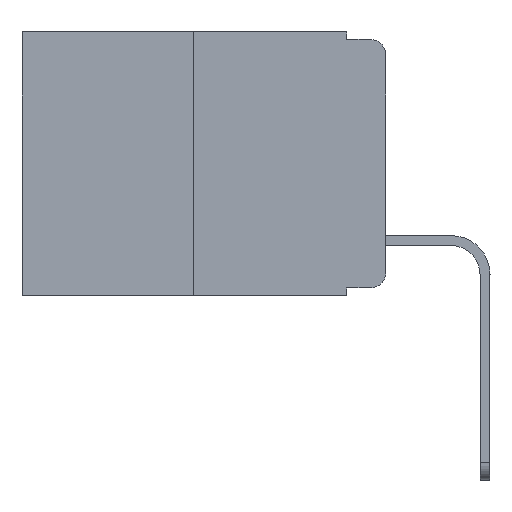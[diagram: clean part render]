
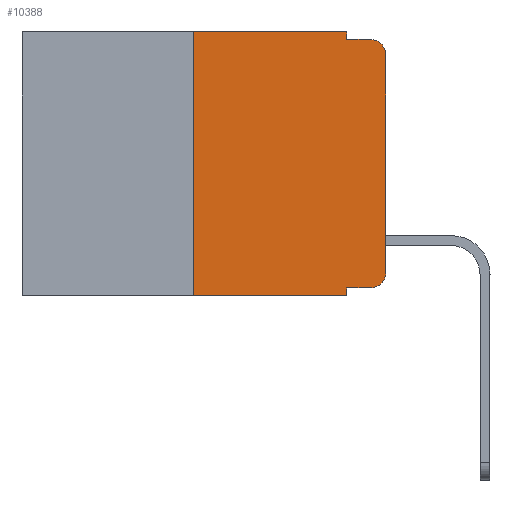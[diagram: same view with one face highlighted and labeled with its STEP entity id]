
A CAD part, left-side view. The second image highlights one B-rep face of the part: STEP entity #10388.
In plain terms, the highlighted planar face has unit normal (-1, 0, 0).
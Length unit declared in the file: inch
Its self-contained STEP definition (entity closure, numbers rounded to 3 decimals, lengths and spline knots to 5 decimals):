
#201 = ORIENTED_EDGE ( 'NONE', *, *, #12562, .F. ) ;
#248 = LINE ( 'NONE', #6495, #12870 ) ;
#377 = VECTOR ( 'NONE', #3629, 39.37008 ) ;
#513 = EDGE_CURVE ( 'NONE', #621, #8496, #1411, .T. ) ;
#551 = CARTESIAN_POINT ( 'NONE',  ( 0., 0.25, 0. ) ) ;
#599 = CARTESIAN_POINT ( 'NONE',  ( 0., 0.051, 0. ) ) ;
#621 = VERTEX_POINT ( 'NONE', #11302 ) ;
#633 = VECTOR ( 'NONE', #8889, 39.37008 ) ;
#639 = DIRECTION ( 'NONE',  ( -1., 0., 0. ) ) ;
#715 = VERTEX_POINT ( 'NONE', #5836 ) ;
#861 = CARTESIAN_POINT ( 'NONE',  ( 0., 0., 0. ) ) ;
#954 = VECTOR ( 'NONE', #7895, 39.37008 ) ;
#1121 = DIRECTION ( 'NONE',  ( 0., -1., 0. ) ) ;
#1175 = EDGE_CURVE ( 'NONE', #5986, #8496, #9322, .T. ) ;
#1293 = ORIENTED_EDGE ( 'NONE', *, *, #5710, .T. ) ;
#1411 = LINE ( 'NONE', #8699, #11864 ) ;
#1932 = ORIENTED_EDGE ( 'NONE', *, *, #1175, .T. ) ;
#2097 = CARTESIAN_POINT ( 'NONE',  ( 0., 0.473, 0. ) ) ;
#2160 = VERTEX_POINT ( 'NONE', #3333 ) ;
#2366 = CARTESIAN_POINT ( 'NONE',  ( 0., 0., -0.03 ) ) ;
#2540 = LINE ( 'NONE', #10883, #633 ) ;
#2688 = VECTOR ( 'NONE', #4903, 39.37008 ) ;
#2716 = LINE ( 'NONE', #7201, #5704 ) ;
#2768 = DIRECTION ( 'NONE',  ( 0., 0., -1. ) ) ;
#2782 = DIRECTION ( 'NONE',  ( 0., 0., -1. ) ) ;
#2850 = ORIENTED_EDGE ( 'NONE', *, *, #10176, .F. ) ;
#2851 = LINE ( 'NONE', #5860, #2688 ) ;
#3039 = PLANE ( 'NONE',  #8041 ) ;
#3333 = CARTESIAN_POINT ( 'NONE',  ( 0., 0., -0.313 ) ) ;
#3343 = ORIENTED_EDGE ( 'NONE', *, *, #513, .F. ) ;
#3537 = VERTEX_POINT ( 'NONE', #551 ) ;
#3629 = DIRECTION ( 'NONE',  ( 0., -1., 0. ) ) ;
#3730 = EDGE_CURVE ( 'NONE', #715, #5687, #9076, .T. ) ;
#4548 = ORIENTED_EDGE ( 'NONE', *, *, #7000, .T. ) ;
#4593 = EDGE_CURVE ( 'NONE', #6780, #12118, #7783, .T. ) ;
#4807 = CARTESIAN_POINT ( 'NONE',  ( 0., 0.051, -0.343 ) ) ;
#4854 = CARTESIAN_POINT ( 'NONE',  ( 0., 0.02, -0.03 ) ) ;
#4892 = FACE_OUTER_BOUND ( 'NONE', #11607, .T. ) ;
#4903 = DIRECTION ( 'NONE',  ( 0., 0., -1. ) ) ;
#5076 = CARTESIAN_POINT ( 'NONE',  ( 0., 0.02, -0.333 ) ) ;
#5303 = EDGE_CURVE ( 'NONE', #6780, #5687, #2716, .T. ) ;
#5468 = AXIS2_PLACEMENT_3D ( 'NONE', #8514, #639, #2768 ) ;
#5687 = VERTEX_POINT ( 'NONE', #4807 ) ;
#5700 = ORIENTED_EDGE ( 'NONE', *, *, #5303, .F. ) ;
#5704 = VECTOR ( 'NONE', #8300, 39.37008 ) ;
#5710 = EDGE_CURVE ( 'NONE', #2160, #5986, #8715, .T. ) ;
#5836 = CARTESIAN_POINT ( 'NONE',  ( 0., 0.25, -0.343 ) ) ;
#5860 = CARTESIAN_POINT ( 'NONE',  ( 0., 0.051, 0. ) ) ;
#5972 = CIRCLE ( 'NONE', #5468, 0.02 ) ;
#5986 = VERTEX_POINT ( 'NONE', #2366 ) ;
#6495 = CARTESIAN_POINT ( 'NONE',  ( 0., 0.25, 0. ) ) ;
#6530 = DIRECTION ( 'NONE',  ( 0., -1., 0. ) ) ;
#6780 = VERTEX_POINT ( 'NONE', #7415 ) ;
#7000 = EDGE_CURVE ( 'NONE', #12118, #2160, #5972, .T. ) ;
#7201 = CARTESIAN_POINT ( 'NONE',  ( 0., 0.051, 0. ) ) ;
#7415 = CARTESIAN_POINT ( 'NONE',  ( 0., 0.051, -0.333 ) ) ;
#7783 = LINE ( 'NONE', #9281, #10146 ) ;
#7895 = DIRECTION ( 'NONE',  ( 0., 0., 1. ) ) ;
#8041 = AXIS2_PLACEMENT_3D ( 'NONE', #2097, #8152, #8242 ) ;
#8152 = DIRECTION ( 'NONE',  ( 1., 0., 0. ) ) ;
#8242 = DIRECTION ( 'NONE',  ( 0., 0., -1. ) ) ;
#8300 = DIRECTION ( 'NONE',  ( 0., 0., -1. ) ) ;
#8496 = VERTEX_POINT ( 'NONE', #10182 ) ;
#8514 = CARTESIAN_POINT ( 'NONE',  ( 0., 0.02, -0.313 ) ) ;
#8657 = CARTESIAN_POINT ( 'NONE',  ( 0., 0.473, -0.343 ) ) ;
#8699 = CARTESIAN_POINT ( 'NONE',  ( 0., 0.051, -0.01 ) ) ;
#8715 = LINE ( 'NONE', #861, #954 ) ;
#8889 = DIRECTION ( 'NONE',  ( 0., -1., 0. ) ) ;
#9076 = LINE ( 'NONE', #8657, #377 ) ;
#9281 = CARTESIAN_POINT ( 'NONE',  ( 0., 0.051, -0.333 ) ) ;
#9322 = CIRCLE ( 'NONE', #9532, 0.02 ) ;
#9532 = AXIS2_PLACEMENT_3D ( 'NONE', #4854, #10814, #2782 ) ;
#9637 = EDGE_CURVE ( 'NONE', #3537, #10764, #2540, .T. ) ;
#10102 = ORIENTED_EDGE ( 'NONE', *, *, #4593, .T. ) ;
#10146 = VECTOR ( 'NONE', #1121, 39.37008 ) ;
#10176 = EDGE_CURVE ( 'NONE', #10764, #621, #2851, .T. ) ;
#10182 = CARTESIAN_POINT ( 'NONE',  ( 0., 0.02, -0.01 ) ) ;
#10388 = ADVANCED_FACE ( 'NONE', ( #4892 ), #3039, .F. ) ;
#10764 = VERTEX_POINT ( 'NONE', #599 ) ;
#10814 = DIRECTION ( 'NONE',  ( -1., 0., 0. ) ) ;
#10883 = CARTESIAN_POINT ( 'NONE',  ( 0., 0.473, 0. ) ) ;
#11302 = CARTESIAN_POINT ( 'NONE',  ( 0., 0.051, -0.01 ) ) ;
#11474 = ORIENTED_EDGE ( 'NONE', *, *, #9637, .F. ) ;
#11607 = EDGE_LOOP ( 'NONE', ( #1293, #1932, #3343, #2850, #11474, #201, #12791, #5700, #10102, #4548 ) ) ;
#11864 = VECTOR ( 'NONE', #6530, 39.37008 ) ;
#12118 = VERTEX_POINT ( 'NONE', #5076 ) ;
#12445 = DIRECTION ( 'NONE',  ( 0., 0., 1. ) ) ;
#12562 = EDGE_CURVE ( 'NONE', #715, #3537, #248, .T. ) ;
#12791 = ORIENTED_EDGE ( 'NONE', *, *, #3730, .T. ) ;
#12870 = VECTOR ( 'NONE', #12445, 39.37008 ) ;
